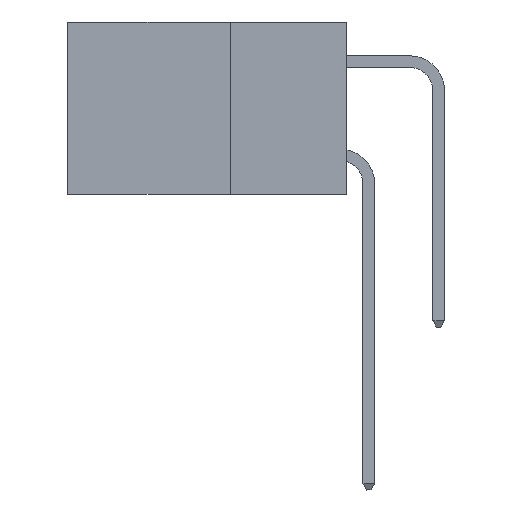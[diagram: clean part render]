
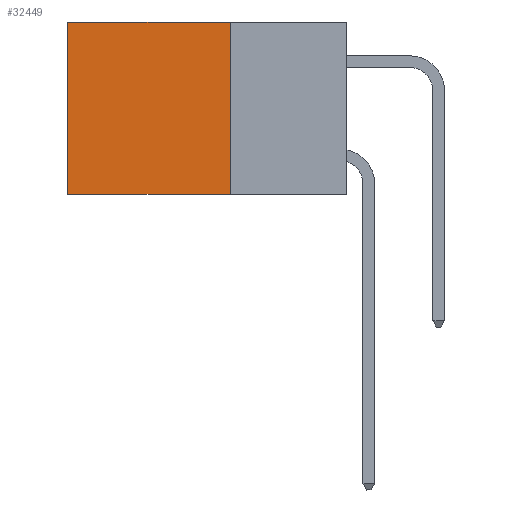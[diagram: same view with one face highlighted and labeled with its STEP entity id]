
A CAD part, left-side view. The second image highlights one B-rep face of the part: STEP entity #32449.
In plain terms, the highlighted planar face has unit normal (-1, 0, 0).
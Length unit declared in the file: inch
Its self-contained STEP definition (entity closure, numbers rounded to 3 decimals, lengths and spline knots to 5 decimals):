
#401 = AXIS2_PLACEMENT_3D ( 'NONE', #29225, #13684, #31797 ) ;
#2621 = LINE ( 'NONE', #31907, #6386 ) ;
#3165 = ORIENTED_EDGE ( 'NONE', *, *, #33426, .F. ) ;
#4029 = ORIENTED_EDGE ( 'NONE', *, *, #6947, .T. ) ;
#4146 = DIRECTION ( 'NONE',  ( 0., 0., -1. ) ) ;
#4247 = DIRECTION ( 'NONE',  ( 0., 0., -1. ) ) ;
#4733 = VECTOR ( 'NONE', #4247, 39.37008 ) ;
#6386 = VECTOR ( 'NONE', #24180, 39.37008 ) ;
#6947 = EDGE_CURVE ( 'NONE', #19982, #31366, #19830, .T. ) ;
#8755 = LINE ( 'NONE', #10781, #21863 ) ;
#9406 = CARTESIAN_POINT ( 'NONE',  ( 0.2875, 0.6, 0. ) ) ;
#10781 = CARTESIAN_POINT ( 'NONE',  ( 0.2875, 0.25, -0.37 ) ) ;
#11809 = LINE ( 'NONE', #20053, #4733 ) ;
#13684 = DIRECTION ( 'NONE',  ( 1., 0., 0. ) ) ;
#13783 = VERTEX_POINT ( 'NONE', #24471 ) ;
#14205 = CARTESIAN_POINT ( 'NONE',  ( 0.2875, 0.6, -0.37 ) ) ;
#16217 = PLANE ( 'NONE',  #401 ) ;
#16630 = EDGE_CURVE ( 'NONE', #13783, #31366, #8755, .T. ) ;
#18069 = CARTESIAN_POINT ( 'NONE',  ( 0.2875, 0.25, 0. ) ) ;
#19260 = FACE_OUTER_BOUND ( 'NONE', #21544, .T. ) ;
#19830 = LINE ( 'NONE', #9406, #27476 ) ;
#19982 = VERTEX_POINT ( 'NONE', #33804 ) ;
#20053 = CARTESIAN_POINT ( 'NONE',  ( 0.2875, 0.25, 0. ) ) ;
#21544 = EDGE_LOOP ( 'NONE', ( #4029, #29451, #3165, #25910 ) ) ;
#21863 = VECTOR ( 'NONE', #31536, 39.37008 ) ;
#24180 = DIRECTION ( 'NONE',  ( 0., 1., 0. ) ) ;
#24471 = CARTESIAN_POINT ( 'NONE',  ( 0.2875, 0.25, -0.37 ) ) ;
#25678 = VERTEX_POINT ( 'NONE', #18069 ) ;
#25910 = ORIENTED_EDGE ( 'NONE', *, *, #27169, .T. ) ;
#27169 = EDGE_CURVE ( 'NONE', #25678, #19982, #2621, .T. ) ;
#27476 = VECTOR ( 'NONE', #4146, 39.37008 ) ;
#29225 = CARTESIAN_POINT ( 'NONE',  ( 0.2875, 0.25, 0. ) ) ;
#29451 = ORIENTED_EDGE ( 'NONE', *, *, #16630, .F. ) ;
#31366 = VERTEX_POINT ( 'NONE', #14205 ) ;
#31536 = DIRECTION ( 'NONE',  ( 0., 1., 0. ) ) ;
#31797 = DIRECTION ( 'NONE',  ( 0., 0., -1. ) ) ;
#31907 = CARTESIAN_POINT ( 'NONE',  ( 0.2875, 0.25, 0. ) ) ;
#32449 = ADVANCED_FACE ( 'NONE', ( #19260 ), #16217, .F. ) ;
#33426 = EDGE_CURVE ( 'NONE', #25678, #13783, #11809, .T. ) ;
#33804 = CARTESIAN_POINT ( 'NONE',  ( 0.2875, 0.6, 0. ) ) ;
